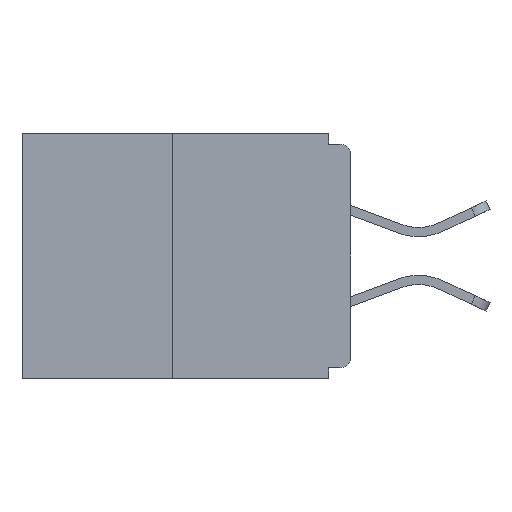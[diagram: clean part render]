
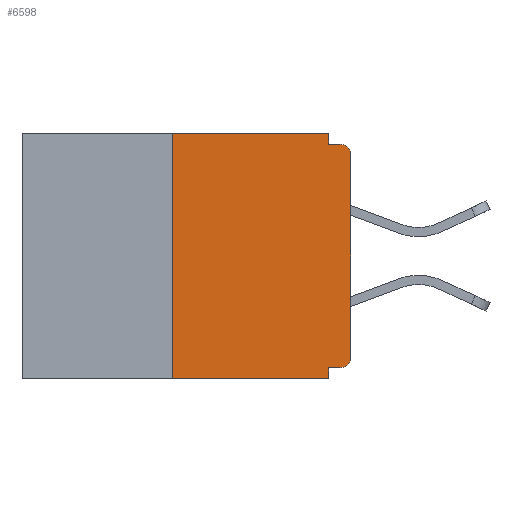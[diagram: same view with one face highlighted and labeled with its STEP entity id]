
A CAD part, left-side view. The second image highlights one B-rep face of the part: STEP entity #6598.
In plain terms, the highlighted planar face has unit normal (-1, 0, 0).
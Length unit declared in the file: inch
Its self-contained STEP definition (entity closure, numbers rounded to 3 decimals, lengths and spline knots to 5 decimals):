
#134 = EDGE_CURVE ( 'NONE', #7734, #3801, #11255, .T. ) ;
#313 = CARTESIAN_POINT ( 'NONE',  ( 0., 0.25, -0.343 ) ) ;
#525 = DIRECTION ( 'NONE',  ( 0., 1., 0. ) ) ;
#662 = ORIENTED_EDGE ( 'NONE', *, *, #9800, .F. ) ;
#1158 = DIRECTION ( 'NONE',  ( -1., 0., 0. ) ) ;
#1274 = CARTESIAN_POINT ( 'NONE',  ( 0., 0.015, -0.03 ) ) ;
#1454 = CARTESIAN_POINT ( 'NONE',  ( 0., 0., -0.03 ) ) ;
#1484 = EDGE_CURVE ( 'NONE', #4150, #7734, #9403, .T. ) ;
#1495 = FACE_OUTER_BOUND ( 'NONE', #4117, .T. ) ;
#1508 = VECTOR ( 'NONE', #6660, 39.37008 ) ;
#1802 = VERTEX_POINT ( 'NONE', #6297 ) ;
#1896 = ORIENTED_EDGE ( 'NONE', *, *, #8761, .T. ) ;
#1963 = CARTESIAN_POINT ( 'NONE',  ( 0., 0.015, -0.313 ) ) ;
#1982 = DIRECTION ( 'NONE',  ( 0., 0., -1. ) ) ;
#2063 = CARTESIAN_POINT ( 'NONE',  ( 0., 0.46, 0. ) ) ;
#2228 = VERTEX_POINT ( 'NONE', #5236 ) ;
#2265 = CARTESIAN_POINT ( 'NONE',  ( 0., 0.46, -0.343 ) ) ;
#2315 = DIRECTION ( 'NONE',  ( 1., 0., 0. ) ) ;
#2347 = DIRECTION ( 'NONE',  ( 0., 0., 1. ) ) ;
#2402 = EDGE_CURVE ( 'NONE', #3860, #8358, #8313, .T. ) ;
#2431 = VECTOR ( 'NONE', #5626, 39.37008 ) ;
#2520 = ORIENTED_EDGE ( 'NONE', *, *, #5145, .F. ) ;
#2690 = AXIS2_PLACEMENT_3D ( 'NONE', #1274, #1158, #1982 ) ;
#2979 = ORIENTED_EDGE ( 'NONE', *, *, #134, .T. ) ;
#3090 = CARTESIAN_POINT ( 'NONE',  ( 0., 0., 0. ) ) ;
#3314 = EDGE_CURVE ( 'NONE', #8358, #1802, #6474, .T. ) ;
#3348 = ORIENTED_EDGE ( 'NONE', *, *, #3791, .F. ) ;
#3400 = VECTOR ( 'NONE', #11414, 39.37008 ) ;
#3761 = DIRECTION ( 'NONE',  ( -1., 0., 0. ) ) ;
#3791 = EDGE_CURVE ( 'NONE', #1802, #3801, #8738, .T. ) ;
#3801 = VERTEX_POINT ( 'NONE', #5820 ) ;
#3827 = ORIENTED_EDGE ( 'NONE', *, *, #3314, .F. ) ;
#3860 = VERTEX_POINT ( 'NONE', #5298 ) ;
#3888 = PLANE ( 'NONE',  #11324 ) ;
#3919 = VECTOR ( 'NONE', #525, 39.37008 ) ;
#3939 = VECTOR ( 'NONE', #7527, 39.37008 ) ;
#3951 = CIRCLE ( 'NONE', #10837, 0.015 ) ;
#3976 = ORIENTED_EDGE ( 'NONE', *, *, #2402, .F. ) ;
#4040 = LINE ( 'NONE', #6720, #8821 ) ;
#4117 = EDGE_LOOP ( 'NONE', ( #3976, #2520, #10715, #11141, #662, #1896, #10523, #2979, #3348, #3827 ) ) ;
#4150 = VERTEX_POINT ( 'NONE', #6744 ) ;
#4480 = DIRECTION ( 'NONE',  ( 0., 0., -1. ) ) ;
#4822 = CARTESIAN_POINT ( 'NONE',  ( 0., 0.46, 0. ) ) ;
#4952 = LINE ( 'NONE', #2265, #3939 ) ;
#5145 = EDGE_CURVE ( 'NONE', #11295, #3860, #6851, .T. ) ;
#5146 = CARTESIAN_POINT ( 'NONE',  ( 0., 0., -0.328 ) ) ;
#5224 = VERTEX_POINT ( 'NONE', #11376 ) ;
#5236 = CARTESIAN_POINT ( 'NONE',  ( 0., 0.031, -0.328 ) ) ;
#5298 = CARTESIAN_POINT ( 'NONE',  ( 0., 0.25, 0. ) ) ;
#5593 = EDGE_CURVE ( 'NONE', #2228, #6260, #4040, .T. ) ;
#5626 = DIRECTION ( 'NONE',  ( 0., -1., 0. ) ) ;
#5659 = DIRECTION ( 'NONE',  ( 0., 0., -1. ) ) ;
#5660 = VECTOR ( 'NONE', #5659, 39.37008 ) ;
#5820 = CARTESIAN_POINT ( 'NONE',  ( 0., 0.015, -0.015 ) ) ;
#5939 = CARTESIAN_POINT ( 'NONE',  ( 0., 0.031, 0. ) ) ;
#6141 = LINE ( 'NONE', #5146, #3919 ) ;
#6260 = VERTEX_POINT ( 'NONE', #7013 ) ;
#6297 = CARTESIAN_POINT ( 'NONE',  ( 0., 0.031, -0.015 ) ) ;
#6474 = LINE ( 'NONE', #10015, #5660 ) ;
#6598 = ADVANCED_FACE ( 'NONE', ( #1495 ), #3888, .F. ) ;
#6660 = DIRECTION ( 'NONE',  ( 0., 0., 1. ) ) ;
#6720 = CARTESIAN_POINT ( 'NONE',  ( 0., 0.031, -0.343 ) ) ;
#6744 = CARTESIAN_POINT ( 'NONE',  ( 0., 0., -0.313 ) ) ;
#6850 = DIRECTION ( 'NONE',  ( 0., 0., -1. ) ) ;
#6851 = LINE ( 'NONE', #8579, #7304 ) ;
#7013 = CARTESIAN_POINT ( 'NONE',  ( 0., 0.031, -0.343 ) ) ;
#7304 = VECTOR ( 'NONE', #2347, 39.37008 ) ;
#7527 = DIRECTION ( 'NONE',  ( 0., -1., 0. ) ) ;
#7734 = VERTEX_POINT ( 'NONE', #1454 ) ;
#7866 = CARTESIAN_POINT ( 'NONE',  ( 0., 0., -0.015 ) ) ;
#8313 = LINE ( 'NONE', #2063, #2431 ) ;
#8358 = VERTEX_POINT ( 'NONE', #5939 ) ;
#8579 = CARTESIAN_POINT ( 'NONE',  ( 0., 0.25, 0. ) ) ;
#8738 = LINE ( 'NONE', #7866, #3400 ) ;
#8761 = EDGE_CURVE ( 'NONE', #5224, #4150, #3951, .T. ) ;
#8821 = VECTOR ( 'NONE', #6850, 39.37008 ) ;
#9403 = LINE ( 'NONE', #3090, #1508 ) ;
#9800 = EDGE_CURVE ( 'NONE', #5224, #2228, #6141, .T. ) ;
#10015 = CARTESIAN_POINT ( 'NONE',  ( 0., 0.031, 0. ) ) ;
#10523 = ORIENTED_EDGE ( 'NONE', *, *, #1484, .T. ) ;
#10532 = EDGE_CURVE ( 'NONE', #11295, #6260, #4952, .T. ) ;
#10715 = ORIENTED_EDGE ( 'NONE', *, *, #10532, .T. ) ;
#10837 = AXIS2_PLACEMENT_3D ( 'NONE', #1963, #3761, #4480 ) ;
#11108 = DIRECTION ( 'NONE',  ( 0., 0., -1. ) ) ;
#11141 = ORIENTED_EDGE ( 'NONE', *, *, #5593, .F. ) ;
#11255 = CIRCLE ( 'NONE', #2690, 0.015 ) ;
#11295 = VERTEX_POINT ( 'NONE', #313 ) ;
#11324 = AXIS2_PLACEMENT_3D ( 'NONE', #4822, #2315, #11108 ) ;
#11376 = CARTESIAN_POINT ( 'NONE',  ( 0., 0.015, -0.328 ) ) ;
#11414 = DIRECTION ( 'NONE',  ( 0., -1., 0. ) ) ;
